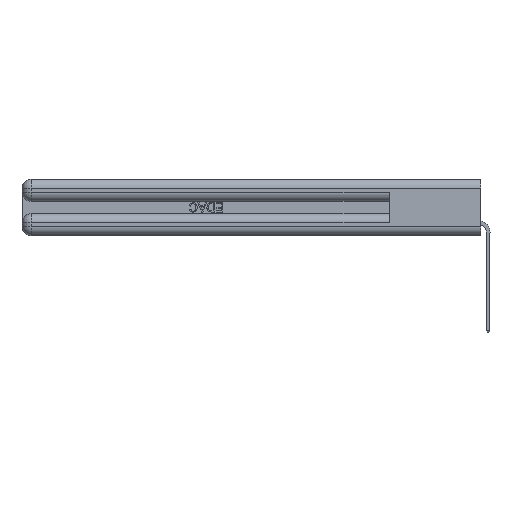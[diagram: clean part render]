
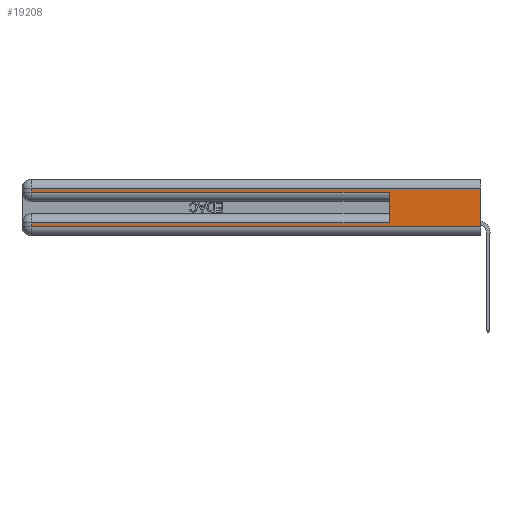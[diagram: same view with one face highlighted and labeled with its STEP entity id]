
A CAD part, left-side view. The second image highlights one B-rep face of the part: STEP entity #19208.
In plain terms, the highlighted planar face has unit normal (-1, 0, 0).
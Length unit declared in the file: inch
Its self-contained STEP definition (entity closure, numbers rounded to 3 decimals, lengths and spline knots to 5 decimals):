
#302 = CARTESIAN_POINT ( 'NONE',  ( 0., 0.6, 0.145 ) ) ;
#457 = VECTOR ( 'NONE', #8000, 39.37008 ) ;
#713 = LINE ( 'NONE', #20316, #21871 ) ;
#1321 = ORIENTED_EDGE ( 'NONE', *, *, #28433, .F. ) ;
#1837 = VECTOR ( 'NONE', #5963, 39.37008 ) ;
#2370 = FACE_OUTER_BOUND ( 'NONE', #4847, .T. ) ;
#3178 = DIRECTION ( 'NONE',  ( 0., 0., -1. ) ) ;
#4087 = EDGE_CURVE ( 'NONE', #32311, #22465, #12874, .T. ) ;
#4501 = LINE ( 'NONE', #25319, #32830 ) ;
#4847 = EDGE_LOOP ( 'NONE', ( #11641, #29360, #35556, #16465, #1321, #15954, #31266, #28451 ) ) ;
#5963 = DIRECTION ( 'NONE',  ( 0., 0., 1. ) ) ;
#7506 = LINE ( 'NONE', #19638, #21363 ) ;
#7543 = CARTESIAN_POINT ( 'NONE',  ( 0., 0., 0.06 ) ) ;
#7556 = VERTEX_POINT ( 'NONE', #26286 ) ;
#7816 = LINE ( 'NONE', #16211, #457 ) ;
#7838 = CARTESIAN_POINT ( 'NONE',  ( 0., 0., 0.31 ) ) ;
#8000 = DIRECTION ( 'NONE',  ( 0., 0., -1. ) ) ;
#9745 = CARTESIAN_POINT ( 'NONE',  ( 0., 0., 0.37 ) ) ;
#10237 = DIRECTION ( 'NONE',  ( 0., 0., -1. ) ) ;
#10566 = EDGE_CURVE ( 'NONE', #24331, #14675, #7506, .T. ) ;
#11641 = ORIENTED_EDGE ( 'NONE', *, *, #12066, .F. ) ;
#12066 = EDGE_CURVE ( 'NONE', #32311, #22872, #7816, .T. ) ;
#12685 = CARTESIAN_POINT ( 'NONE',  ( 0., 0., 0.06 ) ) ;
#12874 = LINE ( 'NONE', #24621, #33042 ) ;
#14675 = VERTEX_POINT ( 'NONE', #33534 ) ;
#15954 = ORIENTED_EDGE ( 'NONE', *, *, #10566, .T. ) ;
#16211 = CARTESIAN_POINT ( 'NONE',  ( 0., 0., 0.37 ) ) ;
#16320 = CARTESIAN_POINT ( 'NONE',  ( 0., 2.94, 0.285 ) ) ;
#16465 = ORIENTED_EDGE ( 'NONE', *, *, #23359, .T. ) ;
#18219 = PLANE ( 'NONE',  #26984 ) ;
#19208 = ADVANCED_FACE ( 'NONE', ( #2370 ), #18219, .F. ) ;
#19638 = CARTESIAN_POINT ( 'NONE',  ( 0., 0., 0.085 ) ) ;
#20316 = CARTESIAN_POINT ( 'NONE',  ( 0., 0., 0.285 ) ) ;
#20489 = DIRECTION ( 'NONE',  ( 0., 0., -1. ) ) ;
#20853 = CARTESIAN_POINT ( 'NONE',  ( 0., 2.94, 0.37 ) ) ;
#21363 = VECTOR ( 'NONE', #23742, 39.37008 ) ;
#21484 = DIRECTION ( 'NONE',  ( 1., 0., 0. ) ) ;
#21871 = VECTOR ( 'NONE', #31289, 39.37008 ) ;
#22427 = VERTEX_POINT ( 'NONE', #29166 ) ;
#22465 = VERTEX_POINT ( 'NONE', #22484 ) ;
#22484 = CARTESIAN_POINT ( 'NONE',  ( 0., 2.94, 0.31 ) ) ;
#22872 = VERTEX_POINT ( 'NONE', #7543 ) ;
#23359 = EDGE_CURVE ( 'NONE', #35054, #7556, #713, .T. ) ;
#23562 = VECTOR ( 'NONE', #32366, 39.37008 ) ;
#23724 = CARTESIAN_POINT ( 'NONE',  ( 0., 0.6, 0.085 ) ) ;
#23742 = DIRECTION ( 'NONE',  ( 0., 1., 0. ) ) ;
#24331 = VERTEX_POINT ( 'NONE', #23724 ) ;
#24386 = EDGE_CURVE ( 'NONE', #22465, #35054, #32912, .T. ) ;
#24621 = CARTESIAN_POINT ( 'NONE',  ( 0., 0., 0.31 ) ) ;
#25319 = CARTESIAN_POINT ( 'NONE',  ( 0., 2.94, 0.37 ) ) ;
#26286 = CARTESIAN_POINT ( 'NONE',  ( 0., 0.6, 0.285 ) ) ;
#26984 = AXIS2_PLACEMENT_3D ( 'NONE', #9745, #21484, #10237 ) ;
#27670 = EDGE_CURVE ( 'NONE', #14675, #22427, #4501, .T. ) ;
#28433 = EDGE_CURVE ( 'NONE', #24331, #7556, #33614, .T. ) ;
#28451 = ORIENTED_EDGE ( 'NONE', *, *, #32234, .T. ) ;
#29066 = VECTOR ( 'NONE', #20489, 39.37008 ) ;
#29166 = CARTESIAN_POINT ( 'NONE',  ( 0., 2.94, 0.06 ) ) ;
#29360 = ORIENTED_EDGE ( 'NONE', *, *, #4087, .T. ) ;
#31266 = ORIENTED_EDGE ( 'NONE', *, *, #27670, .T. ) ;
#31289 = DIRECTION ( 'NONE',  ( 0., -1., 0. ) ) ;
#32132 = DIRECTION ( 'NONE',  ( 0., 1., 0. ) ) ;
#32234 = EDGE_CURVE ( 'NONE', #22427, #22872, #32537, .T. ) ;
#32311 = VERTEX_POINT ( 'NONE', #7838 ) ;
#32366 = DIRECTION ( 'NONE',  ( 0., -1., 0. ) ) ;
#32537 = LINE ( 'NONE', #12685, #23562 ) ;
#32830 = VECTOR ( 'NONE', #3178, 39.37008 ) ;
#32912 = LINE ( 'NONE', #20853, #29066 ) ;
#33042 = VECTOR ( 'NONE', #32132, 39.37008 ) ;
#33534 = CARTESIAN_POINT ( 'NONE',  ( 0., 2.94, 0.085 ) ) ;
#33614 = LINE ( 'NONE', #302, #1837 ) ;
#35054 = VERTEX_POINT ( 'NONE', #16320 ) ;
#35556 = ORIENTED_EDGE ( 'NONE', *, *, #24386, .T. ) ;
